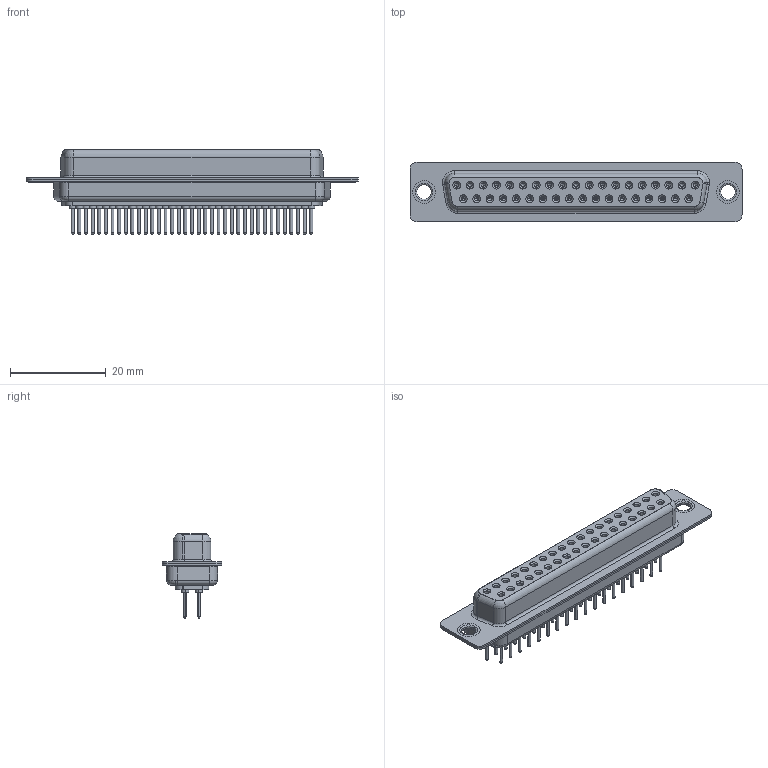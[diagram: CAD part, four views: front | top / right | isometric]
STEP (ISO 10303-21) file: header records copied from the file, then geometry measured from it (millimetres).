
FILE_DESCRIPTION (( 'STEP AP203' ), '1' );
FILE_NAME ('628-M37-221-BN1.STEP', '2020-07-17T03:43:48', ( '' ), ( '' ), 'SwSTEP 2.0', 'SolidWorks 2020', '' );
FILE_SCHEMA (( 'CONFIG_CONTROL_DESIGN' ));
Length unit declared in the file: millimetre
Products named in the file (7): 628M Contact Row 1_21; 628M Contact Row 2_21; 628M Shell Front_37 Contacts; 628M Housing_37 Contacts; 628-M37-221-BN1; 628M Thru Hole Rivet; 628M Shell Rear_37 Contacts
Assembly tree (42 placements, depth 2):
  628-M37-221-BN1
    628M Housing_37 Contacts
    628M Shell Front_37 Contacts
    628M Shell Rear_37 Contacts
    628M Contact Row 1_21  x19
    628M Contact Row 2_21  x18
    628M Thru Hole Rivet  x2
Bounding box: 69.4 x 12.5 x 17.6 mm (x, y, z)
Volume: 5175.2 mm3; surface area: 12520.3 mm2
Topology: 42 solids, 42 shells, 2288 faces, 5265 edges, 3220 vertices
Faces by surface type: cylinder 824, plane 622, torus 583, cone 259
Entity records: 24713 total; most frequent: DIRECTION 4485, CARTESIAN_POINT 3999, ORIENTED_EDGE 3582, AXIS2_PLACEMENT_3D 1912, EDGE_CURVE 1791, VERTEX_POINT 1131, CIRCLE 1069, EDGE_LOOP 1012
